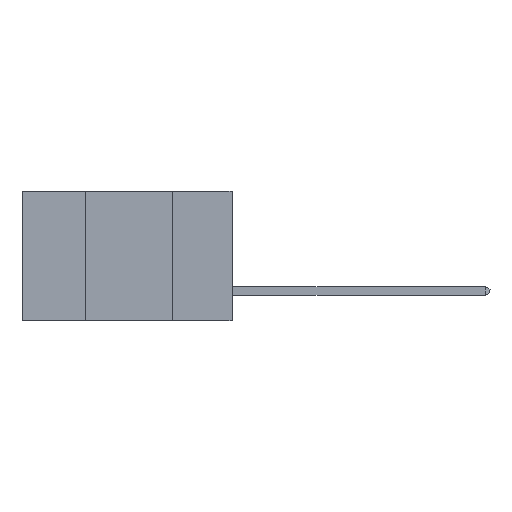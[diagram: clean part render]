
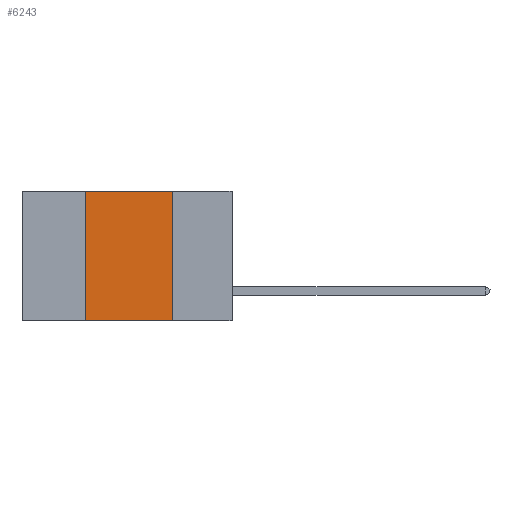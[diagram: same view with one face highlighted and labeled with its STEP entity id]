
A CAD part, left-side view. The second image highlights one B-rep face of the part: STEP entity #6243.
In plain terms, the highlighted planar face has unit normal (-1, 0, 0).
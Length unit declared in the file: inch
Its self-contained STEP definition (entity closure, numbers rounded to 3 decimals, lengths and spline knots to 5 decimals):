
#802 = VECTOR ( 'NONE', #7044, 39.37008 ) ;
#972 = LINE ( 'NONE', #1656, #6741 ) ;
#1347 = ORIENTED_EDGE ( 'NONE', *, *, #10803, .T. ) ;
#1656 = CARTESIAN_POINT ( 'NONE',  ( 0., 0.6, -0.37 ) ) ;
#3350 = ORIENTED_EDGE ( 'NONE', *, *, #8455, .F. ) ;
#3665 = CARTESIAN_POINT ( 'NONE',  ( 0., 0.17, 0. ) ) ;
#3705 = AXIS2_PLACEMENT_3D ( 'NONE', #8534, #10617, #4521 ) ;
#3754 = CARTESIAN_POINT ( 'NONE',  ( 0., 0.42, 0. ) ) ;
#3832 = LINE ( 'NONE', #7162, #802 ) ;
#4118 = FACE_OUTER_BOUND ( 'NONE', #5585, .T. ) ;
#4521 = DIRECTION ( 'NONE',  ( 0., 0., -1. ) ) ;
#4755 = CARTESIAN_POINT ( 'NONE',  ( 0., 0.42, -0.37 ) ) ;
#5129 = DIRECTION ( 'NONE',  ( 0., 0., 1. ) ) ;
#5497 = EDGE_CURVE ( 'NONE', #12631, #11685, #3832, .T. ) ;
#5585 = EDGE_LOOP ( 'NONE', ( #6562, #8824, #3350, #1347 ) ) ;
#6243 = ADVANCED_FACE ( 'NONE', ( #4118 ), #6737, .F. ) ;
#6469 = VECTOR ( 'NONE', #5129, 39.37008 ) ;
#6562 = ORIENTED_EDGE ( 'NONE', *, *, #8219, .F. ) ;
#6737 = PLANE ( 'NONE',  #3705 ) ;
#6741 = VECTOR ( 'NONE', #11851, 39.37008 ) ;
#7044 = DIRECTION ( 'NONE',  ( 0., -1., 0. ) ) ;
#7162 = CARTESIAN_POINT ( 'NONE',  ( 0., 0.6, 0. ) ) ;
#7385 = DIRECTION ( 'NONE',  ( 0., 0., -1. ) ) ;
#8201 = CARTESIAN_POINT ( 'NONE',  ( 0., 0.17, -0.37 ) ) ;
#8219 = EDGE_CURVE ( 'NONE', #11685, #8954, #11734, .T. ) ;
#8376 = CARTESIAN_POINT ( 'NONE',  ( 0., 0.17, 0. ) ) ;
#8455 = EDGE_CURVE ( 'NONE', #12414, #12631, #12871, .T. ) ;
#8534 = CARTESIAN_POINT ( 'NONE',  ( 0., 0.6, 0. ) ) ;
#8824 = ORIENTED_EDGE ( 'NONE', *, *, #5497, .F. ) ;
#8954 = VERTEX_POINT ( 'NONE', #8201 ) ;
#10617 = DIRECTION ( 'NONE',  ( 1., 0., 0. ) ) ;
#10803 = EDGE_CURVE ( 'NONE', #12414, #8954, #972, .T. ) ;
#11260 = CARTESIAN_POINT ( 'NONE',  ( 0., 0.42, 0. ) ) ;
#11685 = VERTEX_POINT ( 'NONE', #3665 ) ;
#11734 = LINE ( 'NONE', #8376, #11908 ) ;
#11851 = DIRECTION ( 'NONE',  ( 0., -1., 0. ) ) ;
#11908 = VECTOR ( 'NONE', #7385, 39.37008 ) ;
#12414 = VERTEX_POINT ( 'NONE', #4755 ) ;
#12631 = VERTEX_POINT ( 'NONE', #11260 ) ;
#12871 = LINE ( 'NONE', #3754, #6469 ) ;
